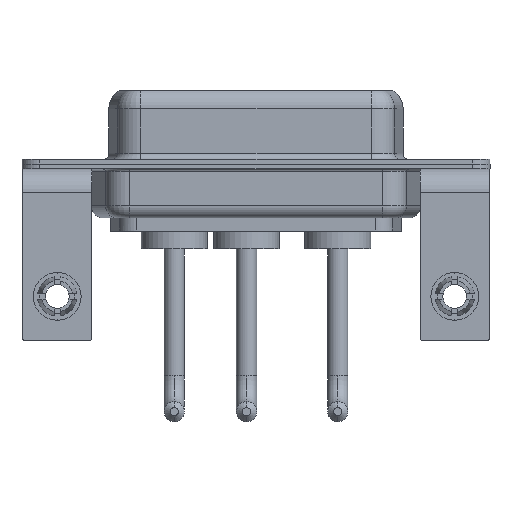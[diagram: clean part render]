
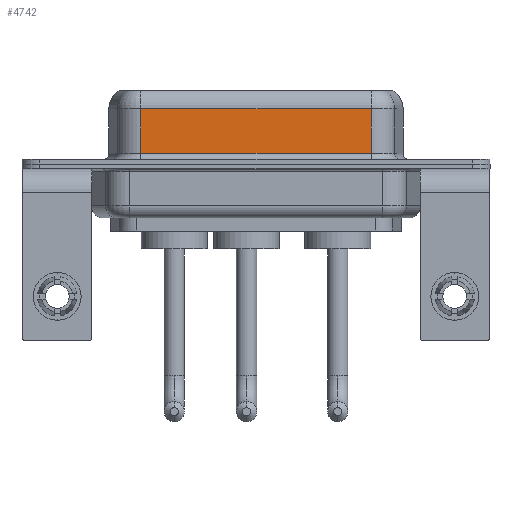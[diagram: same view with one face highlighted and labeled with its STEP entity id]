
A CAD part, front view. The second image highlights one B-rep face of the part: STEP entity #4742.
In plain terms, the highlighted planar face has unit normal (0, -1, 0).
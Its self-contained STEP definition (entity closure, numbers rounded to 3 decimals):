
#409 = EDGE_CURVE ( 'NONE', #10989, #13810, #8680, .T. ) ;
#665 = EDGE_LOOP ( 'NONE', ( #10028, #4512, #12057, #6096 ) ) ;
#724 = CARTESIAN_POINT ( 'NONE',  ( 26.287, -3.95, 4.65 ) ) ;
#1882 = LINE ( 'NONE', #4324, #15917 ) ;
#3055 = CARTESIAN_POINT ( 'NONE',  ( 7.013, -3.95, 6.4 ) ) ;
#3430 = VECTOR ( 'NONE', #5783, 1000. ) ;
#3883 = EDGE_CURVE ( 'NONE', #13810, #6499, #15409, .T. ) ;
#4324 = CARTESIAN_POINT ( 'NONE',  ( 26.287, -3.95, 0.9 ) ) ;
#4450 = CARTESIAN_POINT ( 'NONE',  ( 26.287, -3.95, 0.9 ) ) ;
#4485 = CARTESIAN_POINT ( 'NONE',  ( 7.013, -3.95, 0.9 ) ) ;
#4512 = ORIENTED_EDGE ( 'NONE', *, *, #409, .T. ) ;
#4542 = DIRECTION ( 'NONE',  ( 0., 0., 1. ) ) ;
#4742 = ADVANCED_FACE ( 'NONE', ( #15836 ), #6916, .F. ) ;
#5043 = CARTESIAN_POINT ( 'NONE',  ( 26.287, -3.95, 4.65 ) ) ;
#5783 = DIRECTION ( 'NONE',  ( 0., 0., -1. ) ) ;
#6096 = ORIENTED_EDGE ( 'NONE', *, *, #6506, .T. ) ;
#6499 = VERTEX_POINT ( 'NONE', #4485 ) ;
#6506 = EDGE_CURVE ( 'NONE', #6499, #14459, #1882, .T. ) ;
#6916 = PLANE ( 'NONE',  #9879 ) ;
#8073 = DIRECTION ( 'NONE',  ( 0., 0., -1. ) ) ;
#8176 = LINE ( 'NONE', #12077, #3430 ) ;
#8680 = LINE ( 'NONE', #5043, #13375 ) ;
#9312 = VECTOR ( 'NONE', #8073, 1000. ) ;
#9424 = DIRECTION ( 'NONE',  ( 1., 0., 0. ) ) ;
#9879 = AXIS2_PLACEMENT_3D ( 'NONE', #15745, #10693, #4542 ) ;
#10028 = ORIENTED_EDGE ( 'NONE', *, *, #12641, .F. ) ;
#10693 = DIRECTION ( 'NONE',  ( 0., 1., 0. ) ) ;
#10831 = CARTESIAN_POINT ( 'NONE',  ( 7.013, -3.95, 4.65 ) ) ;
#10989 = VERTEX_POINT ( 'NONE', #724 ) ;
#12057 = ORIENTED_EDGE ( 'NONE', *, *, #3883, .T. ) ;
#12077 = CARTESIAN_POINT ( 'NONE',  ( 26.287, -3.95, 6.4 ) ) ;
#12641 = EDGE_CURVE ( 'NONE', #10989, #14459, #8176, .T. ) ;
#13375 = VECTOR ( 'NONE', #16104, 1000. ) ;
#13810 = VERTEX_POINT ( 'NONE', #10831 ) ;
#14459 = VERTEX_POINT ( 'NONE', #4450 ) ;
#15409 = LINE ( 'NONE', #3055, #9312 ) ;
#15745 = CARTESIAN_POINT ( 'NONE',  ( 26.287, -3.95, 6.4 ) ) ;
#15836 = FACE_OUTER_BOUND ( 'NONE', #665, .T. ) ;
#15917 = VECTOR ( 'NONE', #9424, 1000. ) ;
#16104 = DIRECTION ( 'NONE',  ( -1., 0., 0. ) ) ;
